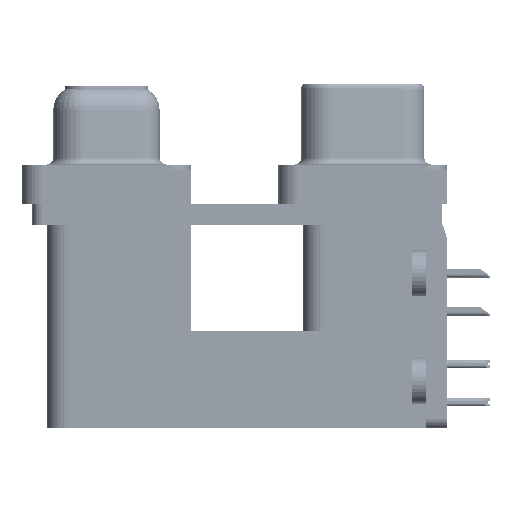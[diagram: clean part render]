
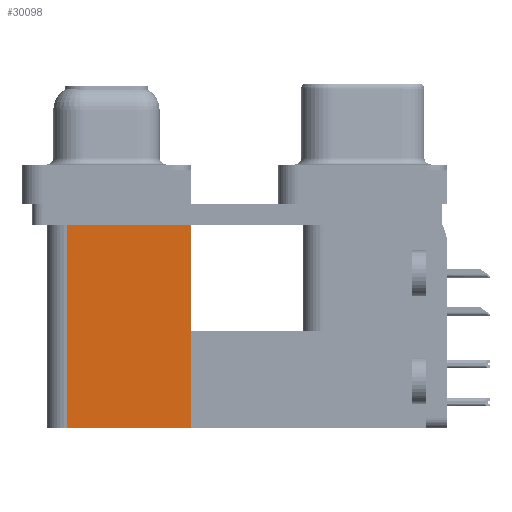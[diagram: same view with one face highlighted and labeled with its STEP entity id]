
A CAD part, left-side view. The second image highlights one B-rep face of the part: STEP entity #30098.
In plain terms, the highlighted planar face has unit normal (-1, 0, 0).
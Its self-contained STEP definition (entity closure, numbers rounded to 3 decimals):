
#2056 = DIRECTION ( 'NONE',  ( 0., 1., 0. ) ) ;
#2271 = DIRECTION ( 'NONE',  ( 0., 0., 1. ) ) ;
#3295 = EDGE_LOOP ( 'NONE', ( #31388, #30512, #37844, #25335 ) ) ;
#3772 = VECTOR ( 'NONE', #10393, 1000. ) ;
#4441 = CARTESIAN_POINT ( 'NONE',  ( 3.7, 21.975, -2.5 ) ) ;
#6220 = LINE ( 'NONE', #40099, #6678 ) ;
#6493 = CARTESIAN_POINT ( 'NONE',  ( 3.7, 12.775, -19.2 ) ) ;
#6678 = VECTOR ( 'NONE', #2056, 1000. ) ;
#9279 = VECTOR ( 'NONE', #44350, 1000. ) ;
#10393 = DIRECTION ( 'NONE',  ( 0., 1., 0. ) ) ;
#15302 = CARTESIAN_POINT ( 'NONE',  ( 3.7, 21.975, -19.2 ) ) ;
#18725 = CARTESIAN_POINT ( 'NONE',  ( 3.7, 12.775, -2.5 ) ) ;
#18799 = LINE ( 'NONE', #48528, #9279 ) ;
#19547 = DIRECTION ( 'NONE',  ( 1., 0., 0. ) ) ;
#20204 = VERTEX_POINT ( 'NONE', #25204 ) ;
#23550 = EDGE_CURVE ( 'NONE', #37051, #44173, #44537, .T. ) ;
#25204 = CARTESIAN_POINT ( 'NONE',  ( 3.7, 21.975, -19.2 ) ) ;
#25335 = ORIENTED_EDGE ( 'NONE', *, *, #43768, .T. ) ;
#25692 = CARTESIAN_POINT ( 'NONE',  ( 3.7, 12.775, -2.5 ) ) ;
#26281 = AXIS2_PLACEMENT_3D ( 'NONE', #6493, #19547, #39852 ) ;
#27605 = PLANE ( 'NONE',  #26281 ) ;
#28984 = EDGE_CURVE ( 'NONE', #52646, #20204, #6220, .T. ) ;
#30098 = ADVANCED_FACE ( 'NONE', ( #44550 ), #27605, .F. ) ;
#30512 = ORIENTED_EDGE ( 'NONE', *, *, #38801, .F. ) ;
#31388 = ORIENTED_EDGE ( 'NONE', *, *, #23550, .T. ) ;
#36761 = CARTESIAN_POINT ( 'NONE',  ( 3.7, 12.775, -19.2 ) ) ;
#37051 = VERTEX_POINT ( 'NONE', #25692 ) ;
#37844 = ORIENTED_EDGE ( 'NONE', *, *, #28984, .F. ) ;
#38801 = EDGE_CURVE ( 'NONE', #20204, #44173, #49219, .T. ) ;
#39852 = DIRECTION ( 'NONE',  ( 0., 0., -1. ) ) ;
#40099 = CARTESIAN_POINT ( 'NONE',  ( 3.7, 12.775, -19.2 ) ) ;
#43768 = EDGE_CURVE ( 'NONE', #52646, #37051, #18799, .T. ) ;
#44173 = VERTEX_POINT ( 'NONE', #4441 ) ;
#44350 = DIRECTION ( 'NONE',  ( 0., 0., 1. ) ) ;
#44537 = LINE ( 'NONE', #18725, #3772 ) ;
#44550 = FACE_OUTER_BOUND ( 'NONE', #3295, .T. ) ;
#47175 = VECTOR ( 'NONE', #2271, 1000. ) ;
#48528 = CARTESIAN_POINT ( 'NONE',  ( 3.7, 12.775, -19.2 ) ) ;
#49219 = LINE ( 'NONE', #15302, #47175 ) ;
#52646 = VERTEX_POINT ( 'NONE', #36761 ) ;
